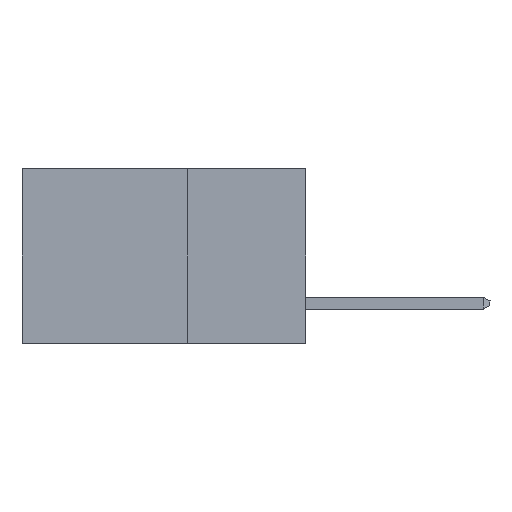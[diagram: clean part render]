
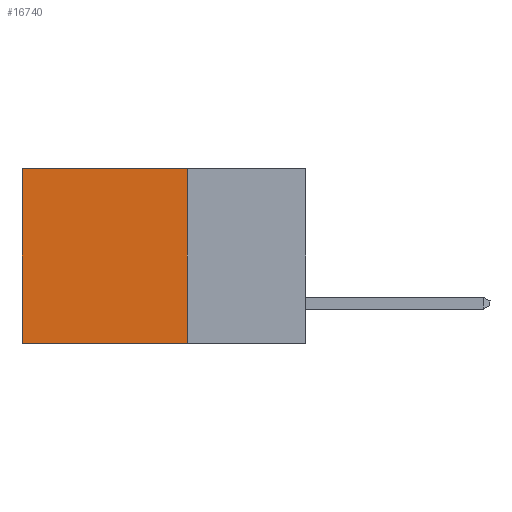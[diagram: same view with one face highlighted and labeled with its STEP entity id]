
A CAD part, left-side view. The second image highlights one B-rep face of the part: STEP entity #16740.
In plain terms, the highlighted planar face has unit normal (-1, 0, 0).
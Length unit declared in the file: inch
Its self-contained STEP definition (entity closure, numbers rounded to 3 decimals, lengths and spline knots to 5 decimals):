
#122 = ORIENTED_EDGE ( 'NONE', *, *, #4300, .F. ) ;
#531 = PLANE ( 'NONE',  #12625 ) ;
#978 = VERTEX_POINT ( 'NONE', #11365 ) ;
#1501 = VECTOR ( 'NONE', #15983, 39.37008 ) ;
#2580 = CARTESIAN_POINT ( 'NONE',  ( 0.298, 0.6, 0. ) ) ;
#2732 = VERTEX_POINT ( 'NONE', #3224 ) ;
#2809 = LINE ( 'NONE', #2580, #6725 ) ;
#2875 = CARTESIAN_POINT ( 'NONE',  ( 0.298, 0.25, 0. ) ) ;
#3224 = CARTESIAN_POINT ( 'NONE',  ( 0.298, 0.25, -0.37 ) ) ;
#3311 = EDGE_CURVE ( 'NONE', #978, #2732, #5488, .T. ) ;
#3942 = EDGE_LOOP ( 'NONE', ( #16511, #122, #7548, #15045 ) ) ;
#4300 = EDGE_CURVE ( 'NONE', #2732, #15390, #10588, .T. ) ;
#4385 = CARTESIAN_POINT ( 'NONE',  ( 0.298, 0.6, 0. ) ) ;
#5488 = LINE ( 'NONE', #14418, #1501 ) ;
#5968 = EDGE_CURVE ( 'NONE', #16975, #15390, #2809, .T. ) ;
#6725 = VECTOR ( 'NONE', #8465, 39.37008 ) ;
#7548 = ORIENTED_EDGE ( 'NONE', *, *, #3311, .F. ) ;
#8465 = DIRECTION ( 'NONE',  ( 0., 0., -1. ) ) ;
#8857 = DIRECTION ( 'NONE',  ( 0., 1., 0. ) ) ;
#10588 = LINE ( 'NONE', #13606, #16774 ) ;
#10846 = LINE ( 'NONE', #2875, #11543 ) ;
#11035 = CARTESIAN_POINT ( 'NONE',  ( 0.298, 0.25, 0. ) ) ;
#11365 = CARTESIAN_POINT ( 'NONE',  ( 0.298, 0.25, 0. ) ) ;
#11543 = VECTOR ( 'NONE', #16787, 39.37008 ) ;
#12551 = DIRECTION ( 'NONE',  ( 0., 0., -1. ) ) ;
#12554 = FACE_OUTER_BOUND ( 'NONE', #3942, .T. ) ;
#12625 = AXIS2_PLACEMENT_3D ( 'NONE', #11035, #15441, #12551 ) ;
#13606 = CARTESIAN_POINT ( 'NONE',  ( 0.298, 0.25, -0.37 ) ) ;
#14418 = CARTESIAN_POINT ( 'NONE',  ( 0.298, 0.25, 0. ) ) ;
#15045 = ORIENTED_EDGE ( 'NONE', *, *, #18699, .T. ) ;
#15390 = VERTEX_POINT ( 'NONE', #19086 ) ;
#15441 = DIRECTION ( 'NONE',  ( 1., 0., 0. ) ) ;
#15983 = DIRECTION ( 'NONE',  ( 0., 0., -1. ) ) ;
#16511 = ORIENTED_EDGE ( 'NONE', *, *, #5968, .T. ) ;
#16740 = ADVANCED_FACE ( 'NONE', ( #12554 ), #531, .F. ) ;
#16774 = VECTOR ( 'NONE', #8857, 39.37008 ) ;
#16787 = DIRECTION ( 'NONE',  ( 0., 1., 0. ) ) ;
#16975 = VERTEX_POINT ( 'NONE', #4385 ) ;
#18699 = EDGE_CURVE ( 'NONE', #978, #16975, #10846, .T. ) ;
#19086 = CARTESIAN_POINT ( 'NONE',  ( 0.298, 0.6, -0.37 ) ) ;
